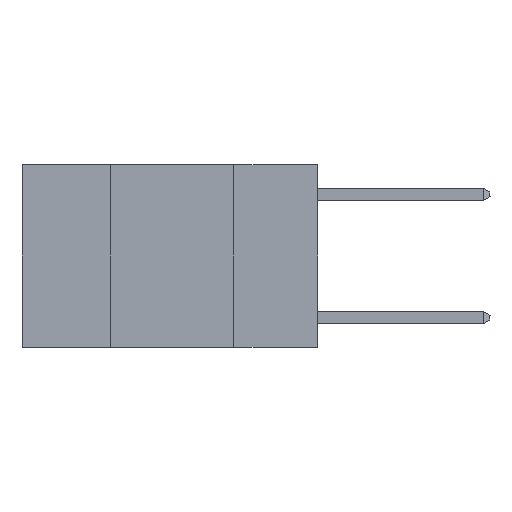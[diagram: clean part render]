
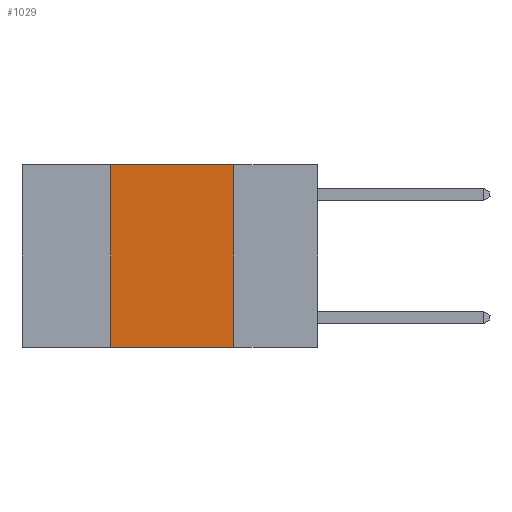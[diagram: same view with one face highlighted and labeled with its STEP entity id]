
A CAD part, left-side view. The second image highlights one B-rep face of the part: STEP entity #1029.
In plain terms, the highlighted planar face has unit normal (-1, 0, 0).
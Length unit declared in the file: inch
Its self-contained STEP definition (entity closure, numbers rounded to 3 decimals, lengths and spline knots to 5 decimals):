
#160 = EDGE_CURVE ( 'NONE', #12254, #9739, #10674, .T. ) ;
#764 = ORIENTED_EDGE ( 'NONE', *, *, #5219, .F. ) ;
#979 = CARTESIAN_POINT ( 'NONE',  ( 0., 0.17, 0. ) ) ;
#1029 = ADVANCED_FACE ( 'NONE', ( #8692 ), #7621, .F. ) ;
#1678 = AXIS2_PLACEMENT_3D ( 'NONE', #6493, #7489, #9840 ) ;
#1859 = CARTESIAN_POINT ( 'NONE',  ( 0., 0.17, -0.37 ) ) ;
#1908 = LINE ( 'NONE', #979, #9159 ) ;
#3816 = ORIENTED_EDGE ( 'NONE', *, *, #160, .F. ) ;
#4381 = DIRECTION ( 'NONE',  ( 0., -1., 0. ) ) ;
#4540 = EDGE_LOOP ( 'NONE', ( #764, #6631, #3816, #5324 ) ) ;
#4844 = CARTESIAN_POINT ( 'NONE',  ( 0., 0.42, 0. ) ) ;
#4859 = VECTOR ( 'NONE', #4381, 39.37008 ) ;
#5122 = DIRECTION ( 'NONE',  ( 0., 0., -1. ) ) ;
#5219 = EDGE_CURVE ( 'NONE', #8673, #9422, #1908, .T. ) ;
#5324 = ORIENTED_EDGE ( 'NONE', *, *, #5804, .T. ) ;
#5804 = EDGE_CURVE ( 'NONE', #12254, #9422, #7811, .T. ) ;
#6250 = VECTOR ( 'NONE', #10811, 39.37008 ) ;
#6493 = CARTESIAN_POINT ( 'NONE',  ( 0., 0.6, 0. ) ) ;
#6631 = ORIENTED_EDGE ( 'NONE', *, *, #9585, .F. ) ;
#7489 = DIRECTION ( 'NONE',  ( 1., 0., 0. ) ) ;
#7621 = PLANE ( 'NONE',  #1678 ) ;
#7811 = LINE ( 'NONE', #14001, #4859 ) ;
#8673 = VERTEX_POINT ( 'NONE', #9893 ) ;
#8692 = FACE_OUTER_BOUND ( 'NONE', #4540, .T. ) ;
#8907 = CARTESIAN_POINT ( 'NONE',  ( 0., 0.6, 0. ) ) ;
#9159 = VECTOR ( 'NONE', #5122, 39.37008 ) ;
#9422 = VERTEX_POINT ( 'NONE', #1859 ) ;
#9585 = EDGE_CURVE ( 'NONE', #9739, #8673, #9836, .T. ) ;
#9739 = VERTEX_POINT ( 'NONE', #4844 ) ;
#9836 = LINE ( 'NONE', #8907, #11256 ) ;
#9840 = DIRECTION ( 'NONE',  ( 0., 0., -1. ) ) ;
#9893 = CARTESIAN_POINT ( 'NONE',  ( 0., 0.17, 0. ) ) ;
#9990 = CARTESIAN_POINT ( 'NONE',  ( 0., 0.42, -0.37 ) ) ;
#10674 = LINE ( 'NONE', #11797, #6250 ) ;
#10811 = DIRECTION ( 'NONE',  ( 0., 0., 1. ) ) ;
#11256 = VECTOR ( 'NONE', #13242, 39.37008 ) ;
#11797 = CARTESIAN_POINT ( 'NONE',  ( 0., 0.42, 0. ) ) ;
#12254 = VERTEX_POINT ( 'NONE', #9990 ) ;
#13242 = DIRECTION ( 'NONE',  ( 0., -1., 0. ) ) ;
#14001 = CARTESIAN_POINT ( 'NONE',  ( 0., 0.6, -0.37 ) ) ;
